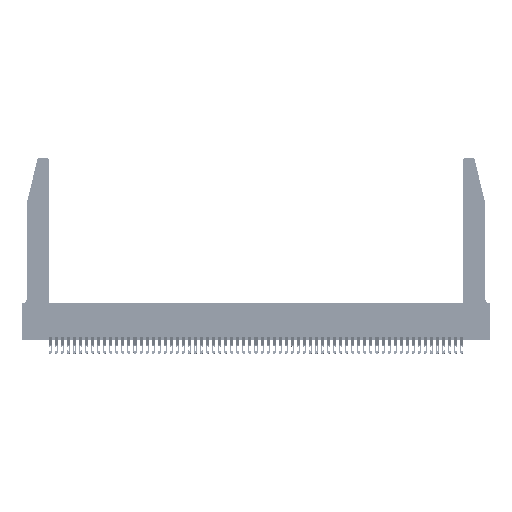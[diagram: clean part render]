
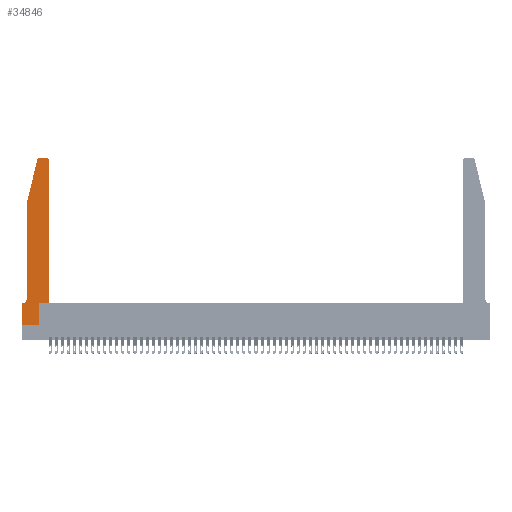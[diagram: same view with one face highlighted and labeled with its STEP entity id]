
A CAD part, top view. The second image highlights one B-rep face of the part: STEP entity #34846.
In plain terms, the highlighted planar face has unit normal (0, 0, 1).
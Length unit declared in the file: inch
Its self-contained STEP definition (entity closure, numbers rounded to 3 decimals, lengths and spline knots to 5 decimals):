
#330 = ORIENTED_EDGE ( 'NONE', *, *, #51488, .T. ) ;
#563 = DIRECTION ( 'NONE',  ( 0., 0., -1. ) ) ;
#1548 = VERTEX_POINT ( 'NONE', #14225 ) ;
#1808 = DIRECTION ( 'NONE',  ( 1., 0., 0. ) ) ;
#2410 = AXIS2_PLACEMENT_3D ( 'NONE', #46496, #41416, #54347 ) ;
#2413 = EDGE_CURVE ( 'NONE', #34268, #4621, #35109, .T. ) ;
#4618 = LINE ( 'NONE', #9445, #23326 ) ;
#4621 = VERTEX_POINT ( 'NONE', #40336 ) ;
#5359 = CARTESIAN_POINT ( 'NONE',  ( 0.4505, 0.35, 0.37 ) ) ;
#5622 = ORIENTED_EDGE ( 'NONE', *, *, #2413, .T. ) ;
#6036 = CARTESIAN_POINT ( 'NONE',  ( 0.4505, 0.35, 0.37 ) ) ;
#6385 = ORIENTED_EDGE ( 'NONE', *, *, #40353, .T. ) ;
#6735 = CIRCLE ( 'NONE', #10614, 0.07 ) ;
#6924 = EDGE_LOOP ( 'NONE', ( #19141, #29298, #6385, #34347, #17310, #48010, #5622, #30752, #48510, #330, #53546, #7307 ) ) ;
#6931 = VECTOR ( 'NONE', #48336, 39.37008 ) ;
#7307 = ORIENTED_EDGE ( 'NONE', *, *, #39187, .T. ) ;
#8238 = VERTEX_POINT ( 'NONE', #49538 ) ;
#8971 = LINE ( 'NONE', #49171, #39916 ) ;
#9445 = CARTESIAN_POINT ( 'NONE',  ( 0.2865, 0.35, 0.37 ) ) ;
#9788 = FACE_OUTER_BOUND ( 'NONE', #6924, .T. ) ;
#10614 = AXIS2_PLACEMENT_3D ( 'NONE', #13322, #563, #34283 ) ;
#10830 = CARTESIAN_POINT ( 'NONE',  ( 0., 0., 0.37 ) ) ;
#11100 = DIRECTION ( 'NONE',  ( 0., 1., 0. ) ) ;
#11248 = VECTOR ( 'NONE', #40918, 39.37008 ) ;
#11977 = LINE ( 'NONE', #51265, #54310 ) ;
#12123 = EDGE_CURVE ( 'NONE', #13840, #17035, #26734, .T. ) ;
#13322 = CARTESIAN_POINT ( 'NONE',  ( 0.0055, 0.42, 0.37 ) ) ;
#13840 = VERTEX_POINT ( 'NONE', #35087 ) ;
#14222 = DIRECTION ( 'NONE',  ( -1., 0., 0. ) ) ;
#14225 = CARTESIAN_POINT ( 'NONE',  ( 0.0755, 0.42, 0.37 ) ) ;
#14352 = VECTOR ( 'NONE', #16218, 39.37008 ) ;
#14586 = EDGE_CURVE ( 'NONE', #19293, #34268, #46844, .T. ) ;
#14811 = CARTESIAN_POINT ( 'NONE',  ( 0., 0.35, 0.37 ) ) ;
#15004 = VECTOR ( 'NONE', #11100, 39.37008 ) ;
#15391 = CARTESIAN_POINT ( 'NONE',  ( 0.25487, 2.72718, 0.37 ) ) ;
#15968 = LINE ( 'NONE', #10830, #11248 ) ;
#16218 = DIRECTION ( 'NONE',  ( 0., -1., 0. ) ) ;
#16622 = CARTESIAN_POINT ( 'NONE',  ( 0., 0.35, 0.37 ) ) ;
#16933 = VERTEX_POINT ( 'NONE', #36161 ) ;
#17035 = VERTEX_POINT ( 'NONE', #15391 ) ;
#17310 = ORIENTED_EDGE ( 'NONE', *, *, #38045, .T. ) ;
#19141 = ORIENTED_EDGE ( 'NONE', *, *, #54423, .T. ) ;
#19293 = VERTEX_POINT ( 'NONE', #43349 ) ;
#19356 = EDGE_CURVE ( 'NONE', #20173, #22263, #27711, .T. ) ;
#20173 = VERTEX_POINT ( 'NONE', #5359 ) ;
#21433 = LINE ( 'NONE', #26431, #34171 ) ;
#21471 = AXIS2_PLACEMENT_3D ( 'NONE', #53266, #40682, #1808 ) ;
#22263 = VERTEX_POINT ( 'NONE', #52642 ) ;
#23326 = VECTOR ( 'NONE', #48008, 39.37008 ) ;
#23737 = DIRECTION ( 'NONE',  ( -0.239, -0.971, 0. ) ) ;
#25996 = AXIS2_PLACEMENT_3D ( 'NONE', #14811, #54042, #49752 ) ;
#26431 = CARTESIAN_POINT ( 'NONE',  ( 0.0755, 2., 0.37 ) ) ;
#26734 = CIRCLE ( 'NONE', #21471, 0.03 ) ;
#27143 = CARTESIAN_POINT ( 'NONE',  ( 0.0755, 0.35, 0.37 ) ) ;
#27711 = LINE ( 'NONE', #32459, #15004 ) ;
#29298 = ORIENTED_EDGE ( 'NONE', *, *, #12123, .T. ) ;
#30752 = ORIENTED_EDGE ( 'NONE', *, *, #54746, .T. ) ;
#32459 = CARTESIAN_POINT ( 'NONE',  ( 0.4505, 0.35, 0.37 ) ) ;
#33131 = EDGE_CURVE ( 'NONE', #8238, #1548, #21433, .T. ) ;
#34171 = VECTOR ( 'NONE', #48466, 39.37008 ) ;
#34268 = VERTEX_POINT ( 'NONE', #16622 ) ;
#34283 = DIRECTION ( 'NONE',  ( -1., 0., 0. ) ) ;
#34347 = ORIENTED_EDGE ( 'NONE', *, *, #33131, .T. ) ;
#34846 = ADVANCED_FACE ( 'NONE', ( #9788 ), #45626, .T. ) ;
#35087 = CARTESIAN_POINT ( 'NONE',  ( 0.284, 2.75, 0.37 ) ) ;
#35109 = LINE ( 'NONE', #41391, #14352 ) ;
#35250 = VECTOR ( 'NONE', #14222, 39.37008 ) ;
#36161 = CARTESIAN_POINT ( 'NONE',  ( 0.2865, 0.35, 0.37 ) ) ;
#37151 = VERTEX_POINT ( 'NONE', #38214 ) ;
#37222 = CIRCLE ( 'NONE', #2410, 0.03 ) ;
#38045 = EDGE_CURVE ( 'NONE', #1548, #19293, #6735, .T. ) ;
#38214 = CARTESIAN_POINT ( 'NONE',  ( 0.2865, 0., 0.37 ) ) ;
#39187 = EDGE_CURVE ( 'NONE', #22263, #42453, #37222, .T. ) ;
#39916 = VECTOR ( 'NONE', #23737, 39.37008 ) ;
#40336 = CARTESIAN_POINT ( 'NONE',  ( 0., 0., 0.37 ) ) ;
#40353 = EDGE_CURVE ( 'NONE', #17035, #8238, #8971, .T. ) ;
#40682 = DIRECTION ( 'NONE',  ( 0., 0., 1. ) ) ;
#40918 = DIRECTION ( 'NONE',  ( 1., 0., 0. ) ) ;
#41391 = CARTESIAN_POINT ( 'NONE',  ( 0., 0., 0.37 ) ) ;
#41416 = DIRECTION ( 'NONE',  ( 0., 0., 1. ) ) ;
#42453 = VERTEX_POINT ( 'NONE', #48477 ) ;
#42824 = DIRECTION ( 'NONE',  ( -1., 0., 0. ) ) ;
#43349 = CARTESIAN_POINT ( 'NONE',  ( 0.0055, 0.35, 0.37 ) ) ;
#43615 = EDGE_CURVE ( 'NONE', #37151, #16933, #4618, .T. ) ;
#45626 = PLANE ( 'NONE',  #25996 ) ;
#46496 = CARTESIAN_POINT ( 'NONE',  ( 0.4205, 2.72, 0.37 ) ) ;
#46844 = LINE ( 'NONE', #27143, #35250 ) ;
#48008 = DIRECTION ( 'NONE',  ( 0., 1., 0. ) ) ;
#48010 = ORIENTED_EDGE ( 'NONE', *, *, #14586, .T. ) ;
#48336 = DIRECTION ( 'NONE',  ( 1., 0., 0. ) ) ;
#48466 = DIRECTION ( 'NONE',  ( 0., -1., 0. ) ) ;
#48477 = CARTESIAN_POINT ( 'NONE',  ( 0.4205, 2.75, 0.37 ) ) ;
#48510 = ORIENTED_EDGE ( 'NONE', *, *, #43615, .T. ) ;
#49171 = CARTESIAN_POINT ( 'NONE',  ( 0.0755, 2., 0.37 ) ) ;
#49538 = CARTESIAN_POINT ( 'NONE',  ( 0.0755, 2., 0.37 ) ) ;
#49752 = DIRECTION ( 'NONE',  ( 1., 0., 0. ) ) ;
#51265 = CARTESIAN_POINT ( 'NONE',  ( 0.2605, 2.75, 0.37 ) ) ;
#51488 = EDGE_CURVE ( 'NONE', #16933, #20173, #52643, .T. ) ;
#52642 = CARTESIAN_POINT ( 'NONE',  ( 0.4505, 2.72, 0.37 ) ) ;
#52643 = LINE ( 'NONE', #6036, #6931 ) ;
#53266 = CARTESIAN_POINT ( 'NONE',  ( 0.284, 2.72, 0.37 ) ) ;
#53546 = ORIENTED_EDGE ( 'NONE', *, *, #19356, .T. ) ;
#54042 = DIRECTION ( 'NONE',  ( 0., 0., 1. ) ) ;
#54310 = VECTOR ( 'NONE', #42824, 39.37008 ) ;
#54347 = DIRECTION ( 'NONE',  ( 1., 0., 0. ) ) ;
#54423 = EDGE_CURVE ( 'NONE', #42453, #13840, #11977, .T. ) ;
#54746 = EDGE_CURVE ( 'NONE', #4621, #37151, #15968, .T. ) ;
